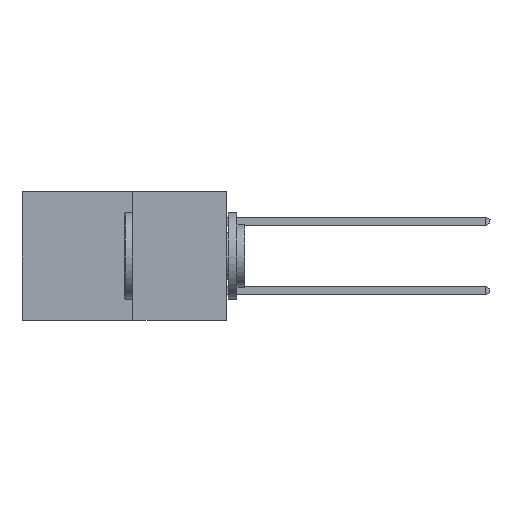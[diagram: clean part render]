
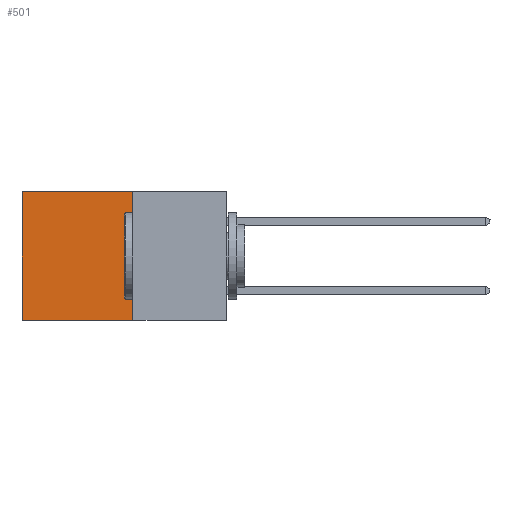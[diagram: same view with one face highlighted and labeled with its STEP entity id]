
A CAD part, left-side view. The second image highlights one B-rep face of the part: STEP entity #501.
In plain terms, the highlighted planar face has unit normal (-1, 0, 0).
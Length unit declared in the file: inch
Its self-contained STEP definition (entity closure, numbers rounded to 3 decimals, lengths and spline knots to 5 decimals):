
#31 = EDGE_CURVE ( 'NONE', #25461, #3302, #27597, .T. ) ;
#501 = ADVANCED_FACE ( 'NONE', ( #26891 ), #8292, .F. ) ;
#516 = VECTOR ( 'NONE', #25112, 39.37008 ) ;
#814 = EDGE_CURVE ( 'NONE', #4012, #17920, #7897, .T. ) ;
#1031 = ORIENTED_EDGE ( 'NONE', *, *, #31, .T. ) ;
#3302 = VERTEX_POINT ( 'NONE', #5654 ) ;
#4012 = VERTEX_POINT ( 'NONE', #25960 ) ;
#5616 = CARTESIAN_POINT ( 'NONE',  ( 0.277, 0.27, 0. ) ) ;
#5654 = CARTESIAN_POINT ( 'NONE',  ( 0.277, 0.59, 0. ) ) ;
#6369 = DIRECTION ( 'NONE',  ( 0., 0., -1. ) ) ;
#7897 = LINE ( 'NONE', #15511, #8605 ) ;
#8292 = PLANE ( 'NONE',  #17379 ) ;
#8605 = VECTOR ( 'NONE', #16037, 39.37008 ) ;
#13336 = CARTESIAN_POINT ( 'NONE',  ( 0.277, 0.27, -0.37 ) ) ;
#13634 = LINE ( 'NONE', #19876, #24903 ) ;
#13786 = EDGE_LOOP ( 'NONE', ( #16970, #26853, #22635, #1031 ) ) ;
#14374 = DIRECTION ( 'NONE',  ( 1., 0., 0. ) ) ;
#15511 = CARTESIAN_POINT ( 'NONE',  ( 0.277, 0.27, -0.37 ) ) ;
#16037 = DIRECTION ( 'NONE',  ( 0., 1., 0. ) ) ;
#16099 = DIRECTION ( 'NONE',  ( 0., 0., -1. ) ) ;
#16115 = CARTESIAN_POINT ( 'NONE',  ( 0.277, 0.59, -0.37 ) ) ;
#16970 = ORIENTED_EDGE ( 'NONE', *, *, #26600, .T. ) ;
#17379 = AXIS2_PLACEMENT_3D ( 'NONE', #13336, #14374, #16099 ) ;
#17920 = VERTEX_POINT ( 'NONE', #16115 ) ;
#18596 = LINE ( 'NONE', #22879, #516 ) ;
#18744 = DIRECTION ( 'NONE',  ( 0., 1., 0. ) ) ;
#19876 = CARTESIAN_POINT ( 'NONE',  ( 0.277, 0.27, -0.37 ) ) ;
#21716 = CARTESIAN_POINT ( 'NONE',  ( 0.277, 0.27, 0. ) ) ;
#21746 = VECTOR ( 'NONE', #18744, 39.37008 ) ;
#22635 = ORIENTED_EDGE ( 'NONE', *, *, #26344, .F. ) ;
#22879 = CARTESIAN_POINT ( 'NONE',  ( 0.277, 0.59, -0.37 ) ) ;
#24903 = VECTOR ( 'NONE', #6369, 39.37008 ) ;
#25112 = DIRECTION ( 'NONE',  ( 0., 0., -1. ) ) ;
#25461 = VERTEX_POINT ( 'NONE', #5616 ) ;
#25960 = CARTESIAN_POINT ( 'NONE',  ( 0.277, 0.27, -0.37 ) ) ;
#26344 = EDGE_CURVE ( 'NONE', #25461, #4012, #13634, .T. ) ;
#26600 = EDGE_CURVE ( 'NONE', #3302, #17920, #18596, .T. ) ;
#26853 = ORIENTED_EDGE ( 'NONE', *, *, #814, .F. ) ;
#26891 = FACE_OUTER_BOUND ( 'NONE', #13786, .T. ) ;
#27597 = LINE ( 'NONE', #21716, #21746 ) ;
